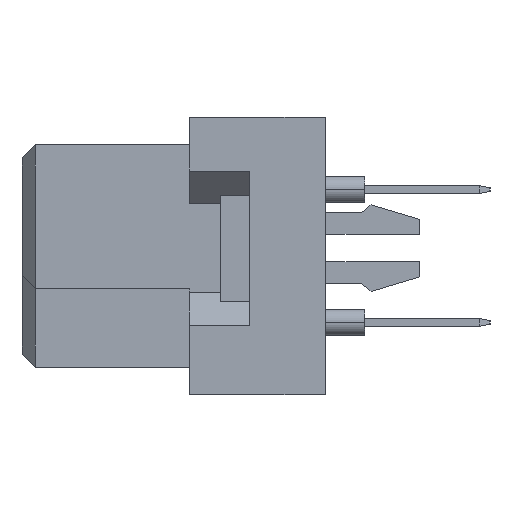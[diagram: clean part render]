
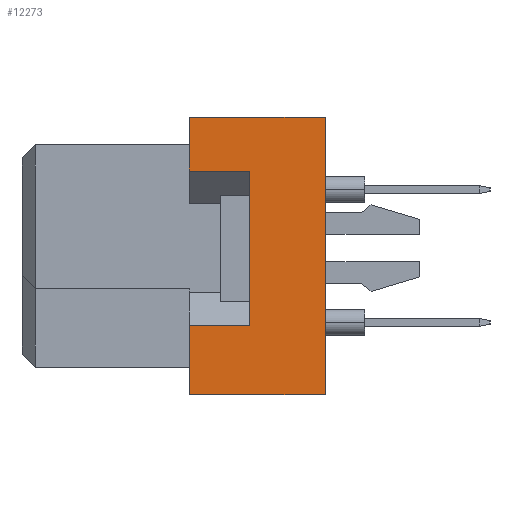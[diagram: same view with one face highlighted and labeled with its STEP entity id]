
A CAD part, left-side view. The second image highlights one B-rep face of the part: STEP entity #12273.
In plain terms, the highlighted planar face has unit normal (-1, 0, 0).
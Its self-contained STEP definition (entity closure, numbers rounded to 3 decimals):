
#228 = DIRECTION ( 'NONE',  ( 0., 1., 0. ) ) ;
#409 = VERTEX_POINT ( 'NONE', #6578 ) ;
#755 = ORIENTED_EDGE ( 'NONE', *, *, #6164, .F. ) ;
#861 = CARTESIAN_POINT ( 'NONE',  ( -27.5, -6.4, -5.3 ) ) ;
#935 = VECTOR ( 'NONE', #16361, 1000. ) ;
#1308 = LINE ( 'NONE', #11413, #935 ) ;
#2503 = LINE ( 'NONE', #15806, #3346 ) ;
#3156 = LINE ( 'NONE', #13049, #19464 ) ;
#3160 = CARTESIAN_POINT ( 'NONE',  ( -27.5, -11.6, -5.3 ) ) ;
#3346 = VECTOR ( 'NONE', #7428, 1000. ) ;
#3690 = VERTEX_POINT ( 'NONE', #9907 ) ;
#3736 = CARTESIAN_POINT ( 'NONE',  ( -27.5, -8.7, 3.25 ) ) ;
#4114 = VECTOR ( 'NONE', #12242, 1000. ) ;
#4785 = LINE ( 'NONE', #3160, #4114 ) ;
#4874 = CARTESIAN_POINT ( 'NONE',  ( -27.5, -11.6, 5.3 ) ) ;
#5201 = VERTEX_POINT ( 'NONE', #18922 ) ;
#6062 = VERTEX_POINT ( 'NONE', #7653 ) ;
#6164 = EDGE_CURVE ( 'NONE', #17173, #3690, #3156, .T. ) ;
#6498 = ORIENTED_EDGE ( 'NONE', *, *, #10467, .F. ) ;
#6578 = CARTESIAN_POINT ( 'NONE',  ( -27.5, -8.7, 3.25 ) ) ;
#7278 = DIRECTION ( 'NONE',  ( 0., 0., 1. ) ) ;
#7428 = DIRECTION ( 'NONE',  ( 0., 1., 0. ) ) ;
#7653 = CARTESIAN_POINT ( 'NONE',  ( -27.5, -8.7, -2.65 ) ) ;
#7794 = FACE_OUTER_BOUND ( 'NONE', #13750, .T. ) ;
#7904 = DIRECTION ( 'NONE',  ( 0., 0., 1. ) ) ;
#7906 = VECTOR ( 'NONE', #7278, 1000. ) ;
#8427 = ORIENTED_EDGE ( 'NONE', *, *, #9315, .T. ) ;
#9063 = ORIENTED_EDGE ( 'NONE', *, *, #15197, .F. ) ;
#9098 = CARTESIAN_POINT ( 'NONE',  ( -27.5, -6.4, 5.3 ) ) ;
#9315 = EDGE_CURVE ( 'NONE', #19935, #20575, #2503, .T. ) ;
#9394 = ORIENTED_EDGE ( 'NONE', *, *, #16028, .F. ) ;
#9437 = ORIENTED_EDGE ( 'NONE', *, *, #19270, .T. ) ;
#9907 = CARTESIAN_POINT ( 'NONE',  ( -27.5, -6.4, -2.65 ) ) ;
#10052 = EDGE_CURVE ( 'NONE', #5201, #19935, #21560, .T. ) ;
#10331 = LINE ( 'NONE', #3736, #16733 ) ;
#10397 = ORIENTED_EDGE ( 'NONE', *, *, #10052, .T. ) ;
#10467 = EDGE_CURVE ( 'NONE', #409, #14233, #10331, .T. ) ;
#11165 = ORIENTED_EDGE ( 'NONE', *, *, #15094, .F. ) ;
#11413 = CARTESIAN_POINT ( 'NONE',  ( -27.5, -8.7, -2.65 ) ) ;
#11581 = CARTESIAN_POINT ( 'NONE',  ( -27.5, -8.7, -2.65 ) ) ;
#11822 = VECTOR ( 'NONE', #19323, 1000. ) ;
#12242 = DIRECTION ( 'NONE',  ( 0., 1., 0. ) ) ;
#12273 = ADVANCED_FACE ( 'NONE', ( #7794 ), #14513, .T. ) ;
#12783 = VECTOR ( 'NONE', #20120, 1000. ) ;
#12881 = CARTESIAN_POINT ( 'NONE',  ( -27.5, -11.6, 5.3 ) ) ;
#13049 = CARTESIAN_POINT ( 'NONE',  ( -27.5, -6.4, -5.3 ) ) ;
#13750 = EDGE_LOOP ( 'NONE', ( #9437, #755, #9394, #10397, #8427, #11165, #6498, #9063 ) ) ;
#14233 = VERTEX_POINT ( 'NONE', #14901 ) ;
#14513 = PLANE ( 'NONE',  #15366 ) ;
#14814 = CARTESIAN_POINT ( 'NONE',  ( -27.5, -6.4, -5.3 ) ) ;
#14901 = CARTESIAN_POINT ( 'NONE',  ( -27.5, -6.4, 3.25 ) ) ;
#14906 = DIRECTION ( 'NONE',  ( 0., 0., 1. ) ) ;
#15094 = EDGE_CURVE ( 'NONE', #14233, #20575, #15922, .T. ) ;
#15197 = EDGE_CURVE ( 'NONE', #6062, #409, #1308, .T. ) ;
#15366 = AXIS2_PLACEMENT_3D ( 'NONE', #12881, #19570, #7904 ) ;
#15806 = CARTESIAN_POINT ( 'NONE',  ( -27.5, -11.6, 5.3 ) ) ;
#15922 = LINE ( 'NONE', #861, #11822 ) ;
#16028 = EDGE_CURVE ( 'NONE', #5201, #17173, #4785, .T. ) ;
#16277 = CARTESIAN_POINT ( 'NONE',  ( -27.5, -11.6, 5.3 ) ) ;
#16361 = DIRECTION ( 'NONE',  ( 0., 0., 1. ) ) ;
#16733 = VECTOR ( 'NONE', #228, 1000. ) ;
#17173 = VERTEX_POINT ( 'NONE', #14814 ) ;
#18922 = CARTESIAN_POINT ( 'NONE',  ( -27.5, -11.6, -5.3 ) ) ;
#19270 = EDGE_CURVE ( 'NONE', #6062, #3690, #19925, .T. ) ;
#19323 = DIRECTION ( 'NONE',  ( 0., 0., 1. ) ) ;
#19464 = VECTOR ( 'NONE', #14906, 1000. ) ;
#19570 = DIRECTION ( 'NONE',  ( -1., 0., 0. ) ) ;
#19925 = LINE ( 'NONE', #11581, #12783 ) ;
#19935 = VERTEX_POINT ( 'NONE', #16277 ) ;
#20120 = DIRECTION ( 'NONE',  ( 0., 1., 0. ) ) ;
#20575 = VERTEX_POINT ( 'NONE', #9098 ) ;
#21560 = LINE ( 'NONE', #4874, #7906 ) ;
